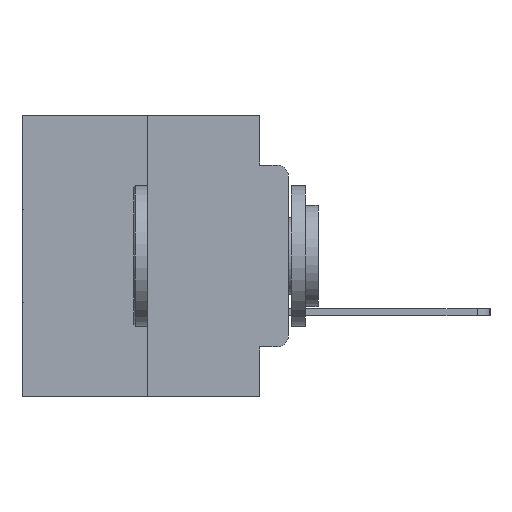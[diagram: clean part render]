
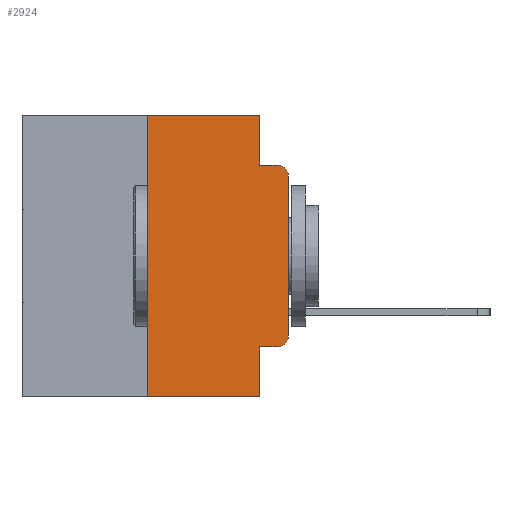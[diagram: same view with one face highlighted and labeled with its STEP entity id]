
A CAD part, left-side view. The second image highlights one B-rep face of the part: STEP entity #2924.
In plain terms, the highlighted planar face has unit normal (-1, 0, 0).
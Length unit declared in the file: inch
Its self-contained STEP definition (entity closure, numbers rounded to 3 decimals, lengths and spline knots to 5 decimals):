
#839 = ORIENTED_EDGE ( 'NONE', *, *, #23131, .T. ) ;
#1131 = EDGE_CURVE ( 'NONE', #14955, #16113, #9126, .T. ) ;
#1382 = CARTESIAN_POINT ( 'NONE',  ( 0., 0.051, -0.4115 ) ) ;
#1992 = DIRECTION ( 'NONE',  ( 0., 0., -1. ) ) ;
#2156 = ORIENTED_EDGE ( 'NONE', *, *, #24637, .F. ) ;
#2200 = ORIENTED_EDGE ( 'NONE', *, *, #1131, .T. ) ;
#2620 = ORIENTED_EDGE ( 'NONE', *, *, #6729, .F. ) ;
#2924 = ADVANCED_FACE ( 'NONE', ( #12948 ), #19242, .F. ) ;
#2979 = EDGE_CURVE ( 'NONE', #16113, #17924, #9956, .T. ) ;
#3313 = ORIENTED_EDGE ( 'NONE', *, *, #20190, .T. ) ;
#3966 = VERTEX_POINT ( 'NONE', #6452 ) ;
#4202 = VECTOR ( 'NONE', #25913, 39.37008 ) ;
#4468 = CARTESIAN_POINT ( 'NONE',  ( 0., 0.25, -0.5 ) ) ;
#5022 = LINE ( 'NONE', #10582, #4202 ) ;
#6063 = CARTESIAN_POINT ( 'NONE',  ( 0., 0.473, 0. ) ) ;
#6083 = VECTOR ( 'NONE', #26845, 39.37008 ) ;
#6210 = VECTOR ( 'NONE', #13995, 39.37008 ) ;
#6452 = CARTESIAN_POINT ( 'NONE',  ( 0., 0.25, 0. ) ) ;
#6729 = EDGE_CURVE ( 'NONE', #3966, #9509, #25122, .T. ) ;
#6871 = VERTEX_POINT ( 'NONE', #26643 ) ;
#6932 = ORIENTED_EDGE ( 'NONE', *, *, #28960, .F. ) ;
#7654 = CARTESIAN_POINT ( 'NONE',  ( 0., 0.051, 0. ) ) ;
#8290 = DIRECTION ( 'NONE',  ( 0., 0., -1. ) ) ;
#9126 = LINE ( 'NONE', #24255, #25230 ) ;
#9317 = EDGE_CURVE ( 'NONE', #24244, #17581, #11957, .T. ) ;
#9509 = VERTEX_POINT ( 'NONE', #7654 ) ;
#9956 = CIRCLE ( 'NONE', #28045, 0.02 ) ;
#10582 = CARTESIAN_POINT ( 'NONE',  ( 0., 0.25, 0. ) ) ;
#10667 = VECTOR ( 'NONE', #16201, 39.37008 ) ;
#10833 = CARTESIAN_POINT ( 'NONE',  ( 0., 0.473, 0. ) ) ;
#11438 = VERTEX_POINT ( 'NONE', #24653 ) ;
#11957 = LINE ( 'NONE', #22450, #6083 ) ;
#12145 = CARTESIAN_POINT ( 'NONE',  ( 0., 0.051, -0.0885 ) ) ;
#12341 = VECTOR ( 'NONE', #18855, 39.37008 ) ;
#12948 = FACE_OUTER_BOUND ( 'NONE', #14513, .T. ) ;
#12986 = DIRECTION ( 'NONE',  ( -1., 0., 0. ) ) ;
#13023 = LINE ( 'NONE', #16521, #12341 ) ;
#13184 = VECTOR ( 'NONE', #14323, 39.37008 ) ;
#13774 = CARTESIAN_POINT ( 'NONE',  ( 0., 0.051, -0.0885 ) ) ;
#13995 = DIRECTION ( 'NONE',  ( 0., 0., -1. ) ) ;
#14323 = DIRECTION ( 'NONE',  ( 0., -1., 0. ) ) ;
#14513 = EDGE_LOOP ( 'NONE', ( #3313, #839, #2156, #19649, #2620, #18316, #28177, #6932, #2200, #27242 ) ) ;
#14955 = VERTEX_POINT ( 'NONE', #1382 ) ;
#15209 = DIRECTION ( 'NONE',  ( 0., -1., 0. ) ) ;
#15357 = CARTESIAN_POINT ( 'NONE',  ( 0., 0., -0.3915 ) ) ;
#15770 = LINE ( 'NONE', #29301, #10667 ) ;
#15791 = DIRECTION ( 'NONE',  ( -1., 0., 0. ) ) ;
#16113 = VERTEX_POINT ( 'NONE', #21195 ) ;
#16201 = DIRECTION ( 'NONE',  ( 0., 0., 1. ) ) ;
#16420 = CARTESIAN_POINT ( 'NONE',  ( 0., 0.051, -0.5 ) ) ;
#16521 = CARTESIAN_POINT ( 'NONE',  ( 0., 0.051, 0. ) ) ;
#17581 = VERTEX_POINT ( 'NONE', #16420 ) ;
#17924 = VERTEX_POINT ( 'NONE', #15357 ) ;
#18316 = ORIENTED_EDGE ( 'NONE', *, *, #27511, .F. ) ;
#18855 = DIRECTION ( 'NONE',  ( 0., 0., -1. ) ) ;
#19242 = PLANE ( 'NONE',  #23681 ) ;
#19272 = VECTOR ( 'NONE', #15209, 39.37008 ) ;
#19649 = ORIENTED_EDGE ( 'NONE', *, *, #26075, .F. ) ;
#20190 = EDGE_CURVE ( 'NONE', #17924, #6871, #15770, .T. ) ;
#20924 = VERTEX_POINT ( 'NONE', #13774 ) ;
#21195 = CARTESIAN_POINT ( 'NONE',  ( 0., 0.02, -0.4115 ) ) ;
#21424 = DIRECTION ( 'NONE',  ( 1., 0., 0. ) ) ;
#22014 = DIRECTION ( 'NONE',  ( 0., -1., 0. ) ) ;
#22450 = CARTESIAN_POINT ( 'NONE',  ( 0., 0.473, -0.5 ) ) ;
#23131 = EDGE_CURVE ( 'NONE', #6871, #11438, #25968, .T. ) ;
#23681 = AXIS2_PLACEMENT_3D ( 'NONE', #6063, #21424, #8290 ) ;
#23774 = LINE ( 'NONE', #29295, #6210 ) ;
#24244 = VERTEX_POINT ( 'NONE', #4468 ) ;
#24255 = CARTESIAN_POINT ( 'NONE',  ( 0., 0.051, -0.4115 ) ) ;
#24637 = EDGE_CURVE ( 'NONE', #20924, #11438, #24904, .T. ) ;
#24653 = CARTESIAN_POINT ( 'NONE',  ( 0., 0.02, -0.0885 ) ) ;
#24904 = LINE ( 'NONE', #12145, #13184 ) ;
#25122 = LINE ( 'NONE', #10833, #19272 ) ;
#25230 = VECTOR ( 'NONE', #22014, 39.37008 ) ;
#25659 = AXIS2_PLACEMENT_3D ( 'NONE', #28904, #15791, #1992 ) ;
#25913 = DIRECTION ( 'NONE',  ( 0., 0., 1. ) ) ;
#25968 = CIRCLE ( 'NONE', #25659, 0.02 ) ;
#26075 = EDGE_CURVE ( 'NONE', #9509, #20924, #23774, .T. ) ;
#26136 = CARTESIAN_POINT ( 'NONE',  ( 0., 0.02, -0.3915 ) ) ;
#26643 = CARTESIAN_POINT ( 'NONE',  ( 0., 0., -0.1085 ) ) ;
#26845 = DIRECTION ( 'NONE',  ( 0., -1., 0. ) ) ;
#27242 = ORIENTED_EDGE ( 'NONE', *, *, #2979, .T. ) ;
#27511 = EDGE_CURVE ( 'NONE', #24244, #3966, #5022, .T. ) ;
#28045 = AXIS2_PLACEMENT_3D ( 'NONE', #26136, #12986, #28291 ) ;
#28177 = ORIENTED_EDGE ( 'NONE', *, *, #9317, .T. ) ;
#28291 = DIRECTION ( 'NONE',  ( 0., 0., -1. ) ) ;
#28904 = CARTESIAN_POINT ( 'NONE',  ( 0., 0.02, -0.1085 ) ) ;
#28960 = EDGE_CURVE ( 'NONE', #14955, #17581, #13023, .T. ) ;
#29295 = CARTESIAN_POINT ( 'NONE',  ( 0., 0.051, 0. ) ) ;
#29301 = CARTESIAN_POINT ( 'NONE',  ( 0., 0., 0. ) ) ;
